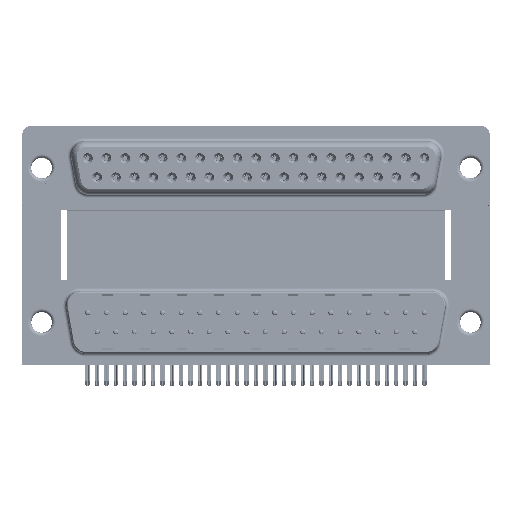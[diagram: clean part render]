
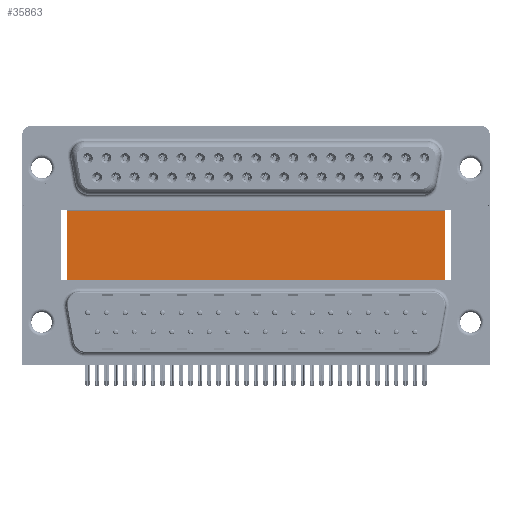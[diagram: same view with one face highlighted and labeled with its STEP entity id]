
A CAD part, top view. The second image highlights one B-rep face of the part: STEP entity #35863.
In plain terms, the highlighted planar face has unit normal (0, 0, 1).
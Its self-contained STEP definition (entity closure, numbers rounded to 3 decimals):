
#887 = VERTEX_POINT ( 'NONE', #67606 ) ;
#1090 = LINE ( 'NONE', #27492, #40424 ) ;
#1208 = VECTOR ( 'NONE', #34476, 1000. ) ;
#3639 = LINE ( 'NONE', #54658, #1208 ) ;
#4436 = LINE ( 'NONE', #66797, #37804 ) ;
#8033 = EDGE_LOOP ( 'NONE', ( #56934, #34657, #65402, #27438 ) ) ;
#9524 = DIRECTION ( 'NONE',  ( 1., 0., 0. ) ) ;
#14628 = PLANE ( 'NONE',  #30776 ) ;
#19185 = DIRECTION ( 'NONE',  ( 0., -1., 0. ) ) ;
#23912 = DIRECTION ( 'NONE',  ( 0., 0., -1. ) ) ;
#25901 = EDGE_CURVE ( 'NONE', #40590, #887, #4436, .T. ) ;
#27335 = CARTESIAN_POINT ( 'NONE',  ( 3.79, 16.585, -12. ) ) ;
#27438 = ORIENTED_EDGE ( 'NONE', *, *, #43400, .T. ) ;
#27492 = CARTESIAN_POINT ( 'NONE',  ( 3.79, -3.735, -12. ) ) ;
#30776 = AXIS2_PLACEMENT_3D ( 'NONE', #40334, #23912, #45452 ) ;
#31825 = EDGE_CURVE ( 'NONE', #40185, #887, #1090, .T. ) ;
#32953 = DIRECTION ( 'NONE',  ( 1., 0., 0. ) ) ;
#34185 = FACE_OUTER_BOUND ( 'NONE', #8033, .T. ) ;
#34476 = DIRECTION ( 'NONE',  ( 0., -1., 0. ) ) ;
#34657 = ORIENTED_EDGE ( 'NONE', *, *, #25901, .F. ) ;
#35255 = CARTESIAN_POINT ( 'NONE',  ( 3.79, 16.585, -12. ) ) ;
#35863 = ADVANCED_FACE ( 'NONE', ( #34185 ), #14628, .F. ) ;
#37804 = VECTOR ( 'NONE', #19185, 1000. ) ;
#40185 = VERTEX_POINT ( 'NONE', #50097 ) ;
#40334 = CARTESIAN_POINT ( 'NONE',  ( 3.79, 16.585, -12. ) ) ;
#40424 = VECTOR ( 'NONE', #32953, 1000. ) ;
#40590 = VERTEX_POINT ( 'NONE', #64421 ) ;
#42364 = EDGE_CURVE ( 'NONE', #42602, #40590, #56464, .T. ) ;
#42602 = VERTEX_POINT ( 'NONE', #27335 ) ;
#43400 = EDGE_CURVE ( 'NONE', #42602, #40185, #3639, .T. ) ;
#45452 = DIRECTION ( 'NONE',  ( -1., 0., 0. ) ) ;
#50097 = CARTESIAN_POINT ( 'NONE',  ( 3.79, -3.735, -12. ) ) ;
#54658 = CARTESIAN_POINT ( 'NONE',  ( 3.79, 16.585, -12. ) ) ;
#56464 = LINE ( 'NONE', #35255, #66961 ) ;
#56934 = ORIENTED_EDGE ( 'NONE', *, *, #31825, .T. ) ;
#64421 = CARTESIAN_POINT ( 'NONE',  ( 59.71, 16.585, -12. ) ) ;
#65402 = ORIENTED_EDGE ( 'NONE', *, *, #42364, .F. ) ;
#66797 = CARTESIAN_POINT ( 'NONE',  ( 59.71, 16.585, -12. ) ) ;
#66961 = VECTOR ( 'NONE', #9524, 1000. ) ;
#67606 = CARTESIAN_POINT ( 'NONE',  ( 59.71, -3.735, -12. ) ) ;
